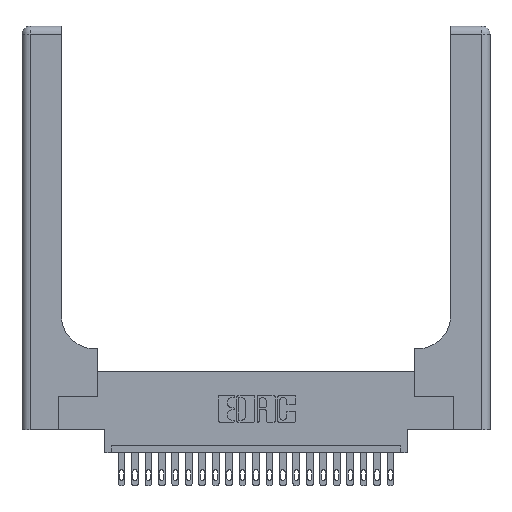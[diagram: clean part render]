
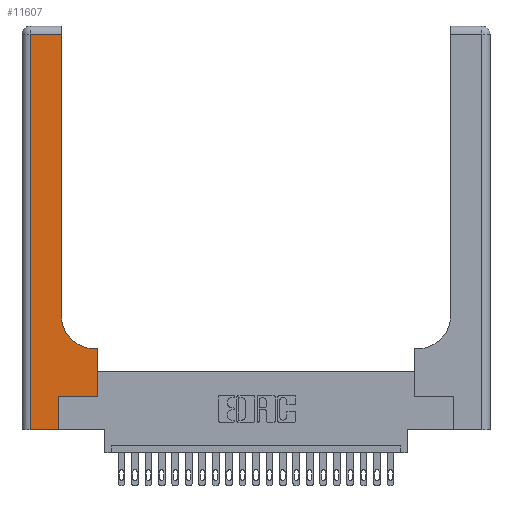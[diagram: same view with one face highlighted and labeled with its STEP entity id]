
A CAD part, top view. The second image highlights one B-rep face of the part: STEP entity #11607.
In plain terms, the highlighted planar face has unit normal (0, 0, 1).
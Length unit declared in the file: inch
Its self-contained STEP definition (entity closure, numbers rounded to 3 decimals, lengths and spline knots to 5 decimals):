
#24 = DIRECTION ( 'NONE',  ( 0., 1., 0. ) ) ;
#198 = VECTOR ( 'NONE', #4751, 39.37008 ) ;
#543 = VERTEX_POINT ( 'NONE', #7162 ) ;
#565 = EDGE_CURVE ( 'NONE', #6867, #11584, #22802, .T. ) ;
#567 = DIRECTION ( 'NONE',  ( 0., 0., -1. ) ) ;
#2136 = CARTESIAN_POINT ( 'NONE',  ( 0.2915, 0.85, 0.37 ) ) ;
#2402 = DIRECTION ( 'NONE',  ( -1., 0., 0. ) ) ;
#3290 = CARTESIAN_POINT ( 'NONE',  ( 0.2915, 2.94, 0.37 ) ) ;
#3500 = LINE ( 'NONE', #20035, #15060 ) ;
#4142 = CARTESIAN_POINT ( 'NONE',  ( 0.269, 0., 0.37 ) ) ;
#4342 = VECTOR ( 'NONE', #11018, 39.37008 ) ;
#4374 = VECTOR ( 'NONE', #4377, 39.37008 ) ;
#4377 = DIRECTION ( 'NONE',  ( 0., 1., 0. ) ) ;
#4751 = DIRECTION ( 'NONE',  ( 0., -1., 0. ) ) ;
#5583 = LINE ( 'NONE', #18223, #19075 ) ;
#6226 = ORIENTED_EDGE ( 'NONE', *, *, #23369, .T. ) ;
#6228 = CARTESIAN_POINT ( 'NONE',  ( 0.06, 3., 0.37 ) ) ;
#6528 = AXIS2_PLACEMENT_3D ( 'NONE', #10353, #14037, #19162 ) ;
#6867 = VERTEX_POINT ( 'NONE', #3290 ) ;
#7162 = CARTESIAN_POINT ( 'NONE',  ( 0.269, 0., 0.37 ) ) ;
#7716 = ORIENTED_EDGE ( 'NONE', *, *, #23533, .T. ) ;
#8134 = CARTESIAN_POINT ( 'NONE',  ( 0.5585, 0.25, 0.37 ) ) ;
#8171 = LINE ( 'NONE', #14948, #14776 ) ;
#8399 = ORIENTED_EDGE ( 'NONE', *, *, #23786, .T. ) ;
#8451 = VERTEX_POINT ( 'NONE', #17752 ) ;
#9090 = DIRECTION ( 'NONE',  ( -1., 0., 0. ) ) ;
#9454 = LINE ( 'NONE', #6228, #198 ) ;
#9866 = CARTESIAN_POINT ( 'NONE',  ( 0.5585, 0.6, 0.37 ) ) ;
#9956 = VERTEX_POINT ( 'NONE', #8134 ) ;
#10353 = CARTESIAN_POINT ( 'NONE',  ( 0.5415, 0.85, 0.37 ) ) ;
#10474 = EDGE_CURVE ( 'NONE', #11584, #22504, #9454, .T. ) ;
#11018 = DIRECTION ( 'NONE',  ( -1., 0., 0. ) ) ;
#11121 = FACE_OUTER_BOUND ( 'NONE', #15739, .T. ) ;
#11537 = PLANE ( 'NONE',  #14284 ) ;
#11584 = VERTEX_POINT ( 'NONE', #16839 ) ;
#11607 = ADVANCED_FACE ( 'NONE', ( #11121 ), #11537, .F. ) ;
#11608 = CARTESIAN_POINT ( 'NONE',  ( 0., 3., 0.37 ) ) ;
#12161 = CARTESIAN_POINT ( 'NONE',  ( 0.2915, 3., 0.37 ) ) ;
#12284 = EDGE_CURVE ( 'NONE', #22504, #543, #14827, .T. ) ;
#12465 = CARTESIAN_POINT ( 'NONE',  ( 0., 2.94, 0.37 ) ) ;
#12755 = LINE ( 'NONE', #4142, #4374 ) ;
#13222 = EDGE_CURVE ( 'NONE', #20647, #17824, #5583, .T. ) ;
#14037 = DIRECTION ( 'NONE',  ( 0., 0., -1. ) ) ;
#14284 = AXIS2_PLACEMENT_3D ( 'NONE', #11608, #567, #2402 ) ;
#14776 = VECTOR ( 'NONE', #24, 39.37008 ) ;
#14827 = LINE ( 'NONE', #18111, #21725 ) ;
#14948 = CARTESIAN_POINT ( 'NONE',  ( 0.5585, 0.25, 0.37 ) ) ;
#15060 = VECTOR ( 'NONE', #23776, 39.37008 ) ;
#15124 = ORIENTED_EDGE ( 'NONE', *, *, #565, .T. ) ;
#15739 = EDGE_LOOP ( 'NONE', ( #16266, #15124, #20334, #15951, #7716, #8399, #6226, #23730, #16982 ) ) ;
#15951 = ORIENTED_EDGE ( 'NONE', *, *, #12284, .T. ) ;
#16107 = VECTOR ( 'NONE', #21400, 39.37008 ) ;
#16145 = EDGE_CURVE ( 'NONE', #17824, #18964, #20884, .T. ) ;
#16266 = ORIENTED_EDGE ( 'NONE', *, *, #20834, .T. ) ;
#16518 = DIRECTION ( 'NONE',  ( 1., 0., 0. ) ) ;
#16839 = CARTESIAN_POINT ( 'NONE',  ( 0.06, 2.94, 0.37 ) ) ;
#16982 = ORIENTED_EDGE ( 'NONE', *, *, #16145, .T. ) ;
#17230 = CARTESIAN_POINT ( 'NONE',  ( 0.06, 0., 0.37 ) ) ;
#17752 = CARTESIAN_POINT ( 'NONE',  ( 0.269, 0.25, 0.37 ) ) ;
#17824 = VERTEX_POINT ( 'NONE', #18357 ) ;
#18111 = CARTESIAN_POINT ( 'NONE',  ( 0., 0., 0.37 ) ) ;
#18223 = CARTESIAN_POINT ( 'NONE',  ( 0.2915, 0.6, 0.37 ) ) ;
#18357 = CARTESIAN_POINT ( 'NONE',  ( 0.5415, 0.6, 0.37 ) ) ;
#18964 = VERTEX_POINT ( 'NONE', #2136 ) ;
#19075 = VECTOR ( 'NONE', #9090, 39.37008 ) ;
#19162 = DIRECTION ( 'NONE',  ( 1., 0., 0. ) ) ;
#19527 = LINE ( 'NONE', #12161, #16107 ) ;
#20035 = CARTESIAN_POINT ( 'NONE',  ( 0.269, 0.25, 0.37 ) ) ;
#20334 = ORIENTED_EDGE ( 'NONE', *, *, #10474, .T. ) ;
#20647 = VERTEX_POINT ( 'NONE', #9866 ) ;
#20834 = EDGE_CURVE ( 'NONE', #18964, #6867, #19527, .T. ) ;
#20884 = CIRCLE ( 'NONE', #6528, 0.25 ) ;
#21400 = DIRECTION ( 'NONE',  ( 0., 1., 0. ) ) ;
#21725 = VECTOR ( 'NONE', #16518, 39.37008 ) ;
#22504 = VERTEX_POINT ( 'NONE', #17230 ) ;
#22802 = LINE ( 'NONE', #12465, #4342 ) ;
#23369 = EDGE_CURVE ( 'NONE', #9956, #20647, #8171, .T. ) ;
#23533 = EDGE_CURVE ( 'NONE', #543, #8451, #12755, .T. ) ;
#23730 = ORIENTED_EDGE ( 'NONE', *, *, #13222, .T. ) ;
#23776 = DIRECTION ( 'NONE',  ( 1., 0., 0. ) ) ;
#23786 = EDGE_CURVE ( 'NONE', #8451, #9956, #3500, .T. ) ;
